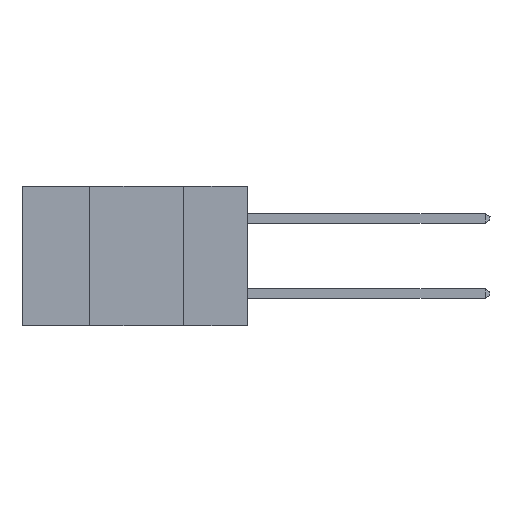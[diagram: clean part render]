
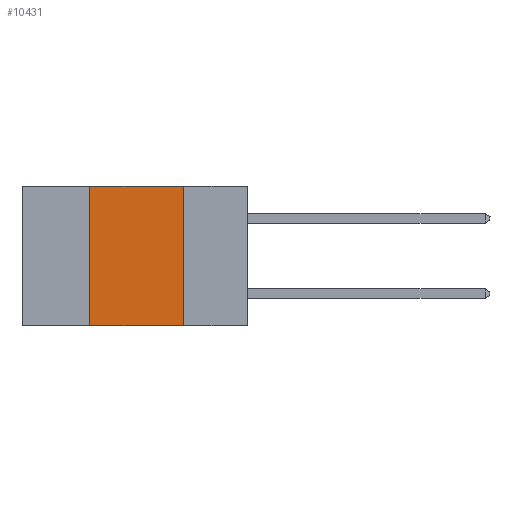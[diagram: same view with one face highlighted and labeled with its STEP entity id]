
A CAD part, left-side view. The second image highlights one B-rep face of the part: STEP entity #10431.
In plain terms, the highlighted planar face has unit normal (-1, 0, 0).
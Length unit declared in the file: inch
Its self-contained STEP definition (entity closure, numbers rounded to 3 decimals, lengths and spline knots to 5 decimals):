
#128 = DIRECTION ( 'NONE',  ( 0., 0., 1. ) ) ;
#162 = VECTOR ( 'NONE', #128, 39.37008 ) ;
#242 = FACE_OUTER_BOUND ( 'NONE', #7368, .T. ) ;
#610 = ORIENTED_EDGE ( 'NONE', *, *, #12188, .F. ) ;
#757 = VECTOR ( 'NONE', #11697, 39.37008 ) ;
#1243 = LINE ( 'NONE', #15724, #2333 ) ;
#1339 = VERTEX_POINT ( 'NONE', #6524 ) ;
#2333 = VECTOR ( 'NONE', #4714, 39.37008 ) ;
#4102 = AXIS2_PLACEMENT_3D ( 'NONE', #9477, #15672, #9327 ) ;
#4193 = VERTEX_POINT ( 'NONE', #14137 ) ;
#4528 = VERTEX_POINT ( 'NONE', #4654 ) ;
#4654 = CARTESIAN_POINT ( 'NONE',  ( 0., 0.42, 0. ) ) ;
#4714 = DIRECTION ( 'NONE',  ( 0., 0., -1. ) ) ;
#5357 = ORIENTED_EDGE ( 'NONE', *, *, #14653, .T. ) ;
#5554 = VERTEX_POINT ( 'NONE', #11909 ) ;
#6388 = LINE ( 'NONE', #10064, #13107 ) ;
#6524 = CARTESIAN_POINT ( 'NONE',  ( 0., 0.17, -0.37 ) ) ;
#6804 = CARTESIAN_POINT ( 'NONE',  ( 0., 0.6, 0. ) ) ;
#7214 = LINE ( 'NONE', #11047, #162 ) ;
#7368 = EDGE_LOOP ( 'NONE', ( #610, #9665, #9473, #5357 ) ) ;
#9004 = PLANE ( 'NONE',  #4102 ) ;
#9327 = DIRECTION ( 'NONE',  ( 0., 0., -1. ) ) ;
#9473 = ORIENTED_EDGE ( 'NONE', *, *, #9644, .F. ) ;
#9477 = CARTESIAN_POINT ( 'NONE',  ( 0., 0.6, 0. ) ) ;
#9644 = EDGE_CURVE ( 'NONE', #5554, #4528, #7214, .T. ) ;
#9665 = ORIENTED_EDGE ( 'NONE', *, *, #13481, .F. ) ;
#10064 = CARTESIAN_POINT ( 'NONE',  ( 0., 0.6, -0.37 ) ) ;
#10431 = ADVANCED_FACE ( 'NONE', ( #242 ), #9004, .F. ) ;
#11047 = CARTESIAN_POINT ( 'NONE',  ( 0., 0.42, -0.37 ) ) ;
#11697 = DIRECTION ( 'NONE',  ( 0., -1., 0. ) ) ;
#11909 = CARTESIAN_POINT ( 'NONE',  ( 0., 0.42, -0.37 ) ) ;
#12188 = EDGE_CURVE ( 'NONE', #4193, #1339, #1243, .T. ) ;
#12907 = LINE ( 'NONE', #6804, #757 ) ;
#13107 = VECTOR ( 'NONE', #14968, 39.37008 ) ;
#13481 = EDGE_CURVE ( 'NONE', #4528, #4193, #12907, .T. ) ;
#14137 = CARTESIAN_POINT ( 'NONE',  ( 0., 0.17, 0. ) ) ;
#14653 = EDGE_CURVE ( 'NONE', #5554, #1339, #6388, .T. ) ;
#14968 = DIRECTION ( 'NONE',  ( 0., -1., 0. ) ) ;
#15672 = DIRECTION ( 'NONE',  ( 1., 0., 0. ) ) ;
#15724 = CARTESIAN_POINT ( 'NONE',  ( 0., 0.17, -0.37 ) ) ;
